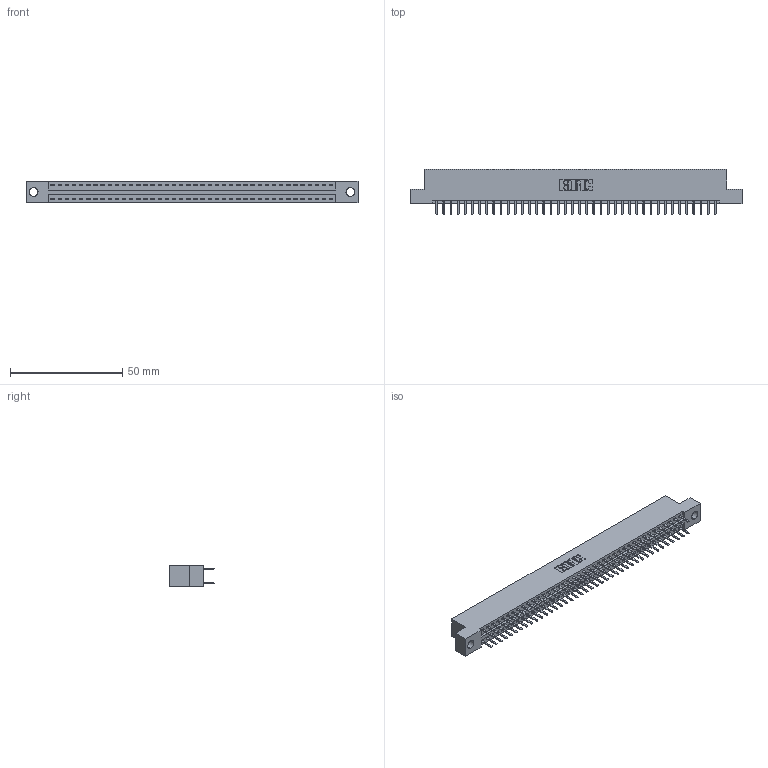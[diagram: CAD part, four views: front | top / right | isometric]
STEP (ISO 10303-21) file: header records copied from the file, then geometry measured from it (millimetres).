
FILE_DESCRIPTION (( 'STEP AP203' ), '1' );
FILE_NAME ('396-080-520-204.STEP', '2019-10-30T22:28:42', ( '' ), ( '' ), 'SwSTEP 2.0', 'SolidWorks 2016', '' );
FILE_SCHEMA (( 'CONFIG_CONTROL_DESIGN' ));
Length unit declared in the file: inch
Products named in the file (3): 396-080-520-204; 345-292-001_345-293-120; 346 Part_Flush Mounting Lugs - 0.156 Dia-TH
Assembly tree (81 placements, depth 2):
  396-080-520-204
    346 Part_Flush Mounting Lugs - 0.156 Dia-TH
    345-292-001_345-293-120  x80
Bounding box: 147.57 x 20.02 x 9.4 mm (x, y, z)
Volume: 14251.7 mm3; surface area: 19289.5 mm2
Topology: 81 solids, 81 shells, 4602 faces, 13369 edges, 8698 vertices
Faces by surface type: plane 3036, cylinder 1566
Entity records: 26491 total; most frequent: CARTESIAN_POINT 4380, ORIENTED_EDGE 4302, DIRECTION 3899, EDGE_CURVE 2151, LINE 1855, VECTOR 1855, VERTEX_POINT 1430, AXIS2_PLACEMENT_3D 1022
